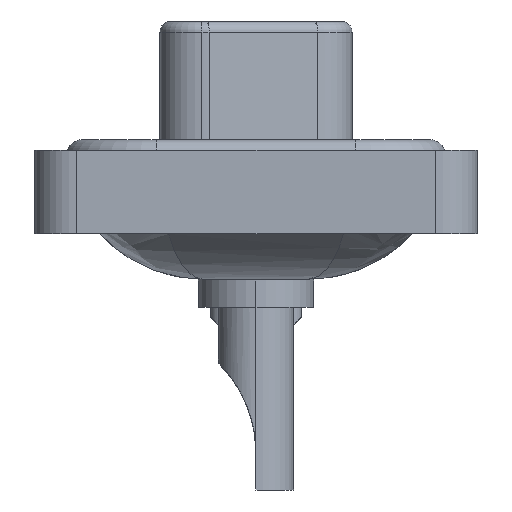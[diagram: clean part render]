
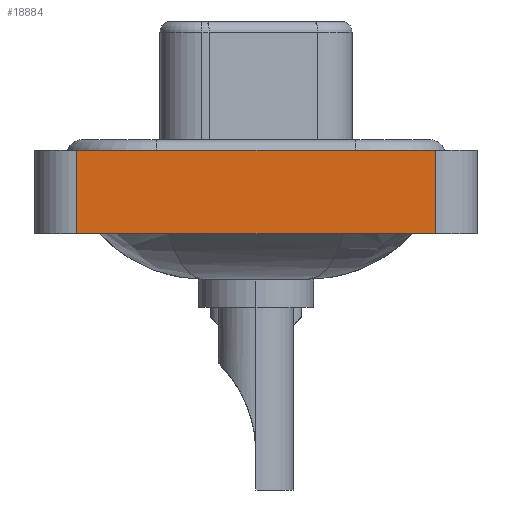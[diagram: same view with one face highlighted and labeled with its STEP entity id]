
A CAD part, left-side view. The second image highlights one B-rep face of the part: STEP entity #18884.
In plain terms, the highlighted planar face has unit normal (-1, 0, 0).
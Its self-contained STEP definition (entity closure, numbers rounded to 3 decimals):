
#374 = VECTOR ( 'NONE', #14805, 1000. ) ;
#471 = VERTEX_POINT ( 'NONE', #16208 ) ;
#534 = EDGE_CURVE ( 'NONE', #19140, #13734, #8436, .T. ) ;
#590 = EDGE_CURVE ( 'NONE', #471, #13734, #5184, .T. ) ;
#648 = CARTESIAN_POINT ( 'NONE',  ( -7.35, -8.55, -3.6 ) ) ;
#919 = LINE ( 'NONE', #2954, #12774 ) ;
#2194 = VECTOR ( 'NONE', #20431, 1000. ) ;
#2360 = DIRECTION ( 'NONE',  ( 0., 0., 1. ) ) ;
#2879 = VECTOR ( 'NONE', #3240, 1000. ) ;
#2954 = CARTESIAN_POINT ( 'NONE',  ( -7.35, -8.55, -3.6 ) ) ;
#3240 = DIRECTION ( 'NONE',  ( 0., -1., 0. ) ) ;
#4265 = DIRECTION ( 'NONE',  ( 0., -1., 0. ) ) ;
#4943 = CARTESIAN_POINT ( 'NONE',  ( -7.35, 8.55, 0.4 ) ) ;
#5184 = LINE ( 'NONE', #648, #2194 ) ;
#5988 = EDGE_CURVE ( 'NONE', #17825, #471, #919, .T. ) ;
#6720 = EDGE_CURVE ( 'NONE', #17825, #19140, #8321, .T. ) ;
#6899 = ORIENTED_EDGE ( 'NONE', *, *, #6720, .F. ) ;
#8223 = CARTESIAN_POINT ( 'NONE',  ( -7.35, 8.55, -3.6 ) ) ;
#8321 = LINE ( 'NONE', #8223, #374 ) ;
#8436 = LINE ( 'NONE', #9855, #2879 ) ;
#9208 = AXIS2_PLACEMENT_3D ( 'NONE', #17513, #10698, #2360 ) ;
#9855 = CARTESIAN_POINT ( 'NONE',  ( -7.35, -8.55, 0.4 ) ) ;
#10698 = DIRECTION ( 'NONE',  ( -1., 0., 0. ) ) ;
#12284 = ORIENTED_EDGE ( 'NONE', *, *, #534, .F. ) ;
#12774 = VECTOR ( 'NONE', #4265, 1000. ) ;
#13734 = VERTEX_POINT ( 'NONE', #14042 ) ;
#14042 = CARTESIAN_POINT ( 'NONE',  ( -7.35, -8.55, 0.4 ) ) ;
#14122 = ORIENTED_EDGE ( 'NONE', *, *, #5988, .T. ) ;
#14492 = ORIENTED_EDGE ( 'NONE', *, *, #590, .T. ) ;
#14805 = DIRECTION ( 'NONE',  ( 0., 0., 1. ) ) ;
#15947 = EDGE_LOOP ( 'NONE', ( #14492, #12284, #6899, #14122 ) ) ;
#16208 = CARTESIAN_POINT ( 'NONE',  ( -7.35, -8.55, -3.6 ) ) ;
#17410 = PLANE ( 'NONE',  #9208 ) ;
#17513 = CARTESIAN_POINT ( 'NONE',  ( -7.35, -8.55, -3.6 ) ) ;
#17825 = VERTEX_POINT ( 'NONE', #18461 ) ;
#18461 = CARTESIAN_POINT ( 'NONE',  ( -7.35, 8.55, -3.6 ) ) ;
#18884 = ADVANCED_FACE ( 'NONE', ( #20748 ), #17410, .T. ) ;
#19140 = VERTEX_POINT ( 'NONE', #4943 ) ;
#20431 = DIRECTION ( 'NONE',  ( 0., 0., 1. ) ) ;
#20748 = FACE_OUTER_BOUND ( 'NONE', #15947, .T. ) ;
